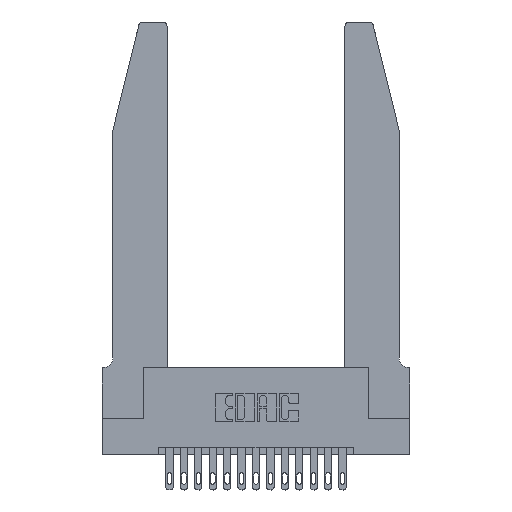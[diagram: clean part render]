
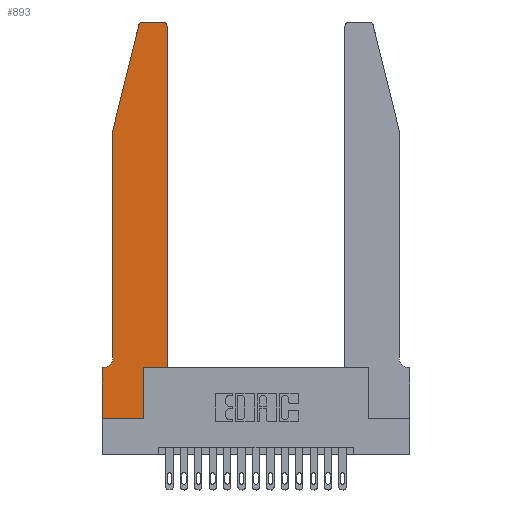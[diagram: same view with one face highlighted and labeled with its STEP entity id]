
A CAD part, top view. The second image highlights one B-rep face of the part: STEP entity #893.
In plain terms, the highlighted planar face has unit normal (0, 0, 1).
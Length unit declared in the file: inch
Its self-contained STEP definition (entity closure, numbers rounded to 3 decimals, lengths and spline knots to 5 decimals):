
#21 = EDGE_CURVE ( 'NONE', #11869, #1695, #6208, .T. ) ;
#676 = LINE ( 'NONE', #16125, #11830 ) ;
#682 = LINE ( 'NONE', #17284, #14336 ) ;
#893 = ADVANCED_FACE ( 'NONE', ( #14101 ), #13317, .T. ) ;
#1071 = EDGE_CURVE ( 'NONE', #3224, #1689, #9797, .T. ) ;
#1089 = LINE ( 'NONE', #2618, #12228 ) ;
#1237 = DIRECTION ( 'NONE',  ( 0., 0., 1. ) ) ;
#1266 = DIRECTION ( 'NONE',  ( -1., 0., 0. ) ) ;
#1309 = VERTEX_POINT ( 'NONE', #16686 ) ;
#1320 = CARTESIAN_POINT ( 'NONE',  ( 0.2865, 0., 0.37 ) ) ;
#1689 = VERTEX_POINT ( 'NONE', #12186 ) ;
#1695 = VERTEX_POINT ( 'NONE', #10525 ) ;
#1908 = ORIENTED_EDGE ( 'NONE', *, *, #2524, .T. ) ;
#2524 = EDGE_CURVE ( 'NONE', #1309, #9897, #1089, .T. ) ;
#2617 = EDGE_CURVE ( 'NONE', #15138, #11822, #16069, .T. ) ;
#2618 = CARTESIAN_POINT ( 'NONE',  ( 0.4505, 0.35, 0.37 ) ) ;
#2886 = VECTOR ( 'NONE', #10107, 39.37008 ) ;
#2991 = CARTESIAN_POINT ( 'NONE',  ( 0.4505, 0.35, 0.37 ) ) ;
#3032 = ORIENTED_EDGE ( 'NONE', *, *, #14612, .T. ) ;
#3224 = VERTEX_POINT ( 'NONE', #11714 ) ;
#3293 = VECTOR ( 'NONE', #7868, 39.37008 ) ;
#3381 = DIRECTION ( 'NONE',  ( 0., 0., 1. ) ) ;
#3836 = EDGE_CURVE ( 'NONE', #9897, #15138, #10806, .T. ) ;
#3841 = EDGE_CURVE ( 'NONE', #11676, #11869, #8314, .T. ) ;
#3956 = CARTESIAN_POINT ( 'NONE',  ( 0.2605, 2.75, 0.37 ) ) ;
#4346 = VERTEX_POINT ( 'NONE', #6788 ) ;
#4356 = CARTESIAN_POINT ( 'NONE',  ( 0.0055, 0.42, 0.37 ) ) ;
#5169 = CARTESIAN_POINT ( 'NONE',  ( 0.0755, 2., 0.37 ) ) ;
#5445 = ORIENTED_EDGE ( 'NONE', *, *, #11831, .T. ) ;
#5540 = DIRECTION ( 'NONE',  ( 1., 0., 0. ) ) ;
#5554 = DIRECTION ( 'NONE',  ( 0., -1., 0. ) ) ;
#5788 = AXIS2_PLACEMENT_3D ( 'NONE', #11943, #3381, #10596 ) ;
#5936 = VECTOR ( 'NONE', #10603, 39.37008 ) ;
#6208 = CIRCLE ( 'NONE', #13917, 0.07 ) ;
#6650 = CARTESIAN_POINT ( 'NONE',  ( 0.0755, 2., 0.37 ) ) ;
#6704 = EDGE_LOOP ( 'NONE', ( #5445, #10141, #14673, #13111, #17718, #12790, #18360, #12419, #3032, #1908, #17313, #9536 ) ) ;
#6788 = CARTESIAN_POINT ( 'NONE',  ( 0.284, 2.75, 0.37 ) ) ;
#7584 = DIRECTION ( 'NONE',  ( 1., 0., 0. ) ) ;
#7868 = DIRECTION ( 'NONE',  ( 0., 1., 0. ) ) ;
#7995 = DIRECTION ( 'NONE',  ( -0.239, -0.971, 0. ) ) ;
#8314 = LINE ( 'NONE', #18711, #11060 ) ;
#8891 = DIRECTION ( 'NONE',  ( 1., 0., 0. ) ) ;
#9236 = EDGE_CURVE ( 'NONE', #17259, #11676, #10289, .T. ) ;
#9365 = VECTOR ( 'NONE', #7995, 39.37008 ) ;
#9536 = ORIENTED_EDGE ( 'NONE', *, *, #2617, .T. ) ;
#9797 = LINE ( 'NONE', #16319, #5936 ) ;
#9897 = VERTEX_POINT ( 'NONE', #2991 ) ;
#9936 = VERTEX_POINT ( 'NONE', #1320 ) ;
#10107 = DIRECTION ( 'NONE',  ( 0., 1., 0. ) ) ;
#10141 = ORIENTED_EDGE ( 'NONE', *, *, #15587, .T. ) ;
#10289 = LINE ( 'NONE', #5169, #9365 ) ;
#10404 = DIRECTION ( 'NONE',  ( 0., 0., 1. ) ) ;
#10525 = CARTESIAN_POINT ( 'NONE',  ( 0.0055, 0.35, 0.37 ) ) ;
#10537 = CARTESIAN_POINT ( 'NONE',  ( 0.4505, 2.72, 0.37 ) ) ;
#10596 = DIRECTION ( 'NONE',  ( 1., 0., 0. ) ) ;
#10603 = DIRECTION ( 'NONE',  ( 0., -1., 0. ) ) ;
#10806 = LINE ( 'NONE', #11510, #2886 ) ;
#11017 = EDGE_CURVE ( 'NONE', #1695, #3224, #682, .T. ) ;
#11060 = VECTOR ( 'NONE', #5554, 39.37008 ) ;
#11303 = CARTESIAN_POINT ( 'NONE',  ( 0.4205, 2.75, 0.37 ) ) ;
#11510 = CARTESIAN_POINT ( 'NONE',  ( 0.4505, 0.35, 0.37 ) ) ;
#11676 = VERTEX_POINT ( 'NONE', #6650 ) ;
#11714 = CARTESIAN_POINT ( 'NONE',  ( 0., 0.35, 0.37 ) ) ;
#11822 = VERTEX_POINT ( 'NONE', #11303 ) ;
#11830 = VECTOR ( 'NONE', #8891, 39.37008 ) ;
#11831 = EDGE_CURVE ( 'NONE', #11822, #4346, #12698, .T. ) ;
#11869 = VERTEX_POINT ( 'NONE', #12575 ) ;
#11943 = CARTESIAN_POINT ( 'NONE',  ( 0., 0.35, 0.37 ) ) ;
#12186 = CARTESIAN_POINT ( 'NONE',  ( 0., 0., 0.37 ) ) ;
#12228 = VECTOR ( 'NONE', #5540, 39.37008 ) ;
#12419 = ORIENTED_EDGE ( 'NONE', *, *, #16807, .T. ) ;
#12575 = CARTESIAN_POINT ( 'NONE',  ( 0.0755, 0.42, 0.37 ) ) ;
#12698 = LINE ( 'NONE', #3956, #12942 ) ;
#12790 = ORIENTED_EDGE ( 'NONE', *, *, #11017, .T. ) ;
#12942 = VECTOR ( 'NONE', #14205, 39.37008 ) ;
#13111 = ORIENTED_EDGE ( 'NONE', *, *, #3841, .T. ) ;
#13317 = PLANE ( 'NONE',  #5788 ) ;
#13917 = AXIS2_PLACEMENT_3D ( 'NONE', #4356, #17276, #18707 ) ;
#14101 = FACE_OUTER_BOUND ( 'NONE', #6704, .T. ) ;
#14205 = DIRECTION ( 'NONE',  ( -1., 0., 0. ) ) ;
#14336 = VECTOR ( 'NONE', #1266, 39.37008 ) ;
#14352 = CARTESIAN_POINT ( 'NONE',  ( 0.4205, 2.72, 0.37 ) ) ;
#14388 = CIRCLE ( 'NONE', #14702, 0.03 ) ;
#14612 = EDGE_CURVE ( 'NONE', #9936, #1309, #17141, .T. ) ;
#14673 = ORIENTED_EDGE ( 'NONE', *, *, #9236, .T. ) ;
#14702 = AXIS2_PLACEMENT_3D ( 'NONE', #17379, #1237, #17260 ) ;
#15138 = VERTEX_POINT ( 'NONE', #10537 ) ;
#15450 = CARTESIAN_POINT ( 'NONE',  ( 0.25487, 2.72718, 0.37 ) ) ;
#15539 = AXIS2_PLACEMENT_3D ( 'NONE', #14352, #10404, #7584 ) ;
#15587 = EDGE_CURVE ( 'NONE', #4346, #17259, #14388, .T. ) ;
#16069 = CIRCLE ( 'NONE', #15539, 0.03 ) ;
#16125 = CARTESIAN_POINT ( 'NONE',  ( 0., 0., 0.37 ) ) ;
#16319 = CARTESIAN_POINT ( 'NONE',  ( 0., 0., 0.37 ) ) ;
#16686 = CARTESIAN_POINT ( 'NONE',  ( 0.2865, 0.35, 0.37 ) ) ;
#16807 = EDGE_CURVE ( 'NONE', #1689, #9936, #676, .T. ) ;
#17141 = LINE ( 'NONE', #17979, #3293 ) ;
#17259 = VERTEX_POINT ( 'NONE', #15450 ) ;
#17260 = DIRECTION ( 'NONE',  ( 1., 0., 0. ) ) ;
#17276 = DIRECTION ( 'NONE',  ( 0., 0., -1. ) ) ;
#17284 = CARTESIAN_POINT ( 'NONE',  ( 0.0755, 0.35, 0.37 ) ) ;
#17313 = ORIENTED_EDGE ( 'NONE', *, *, #3836, .T. ) ;
#17379 = CARTESIAN_POINT ( 'NONE',  ( 0.284, 2.72, 0.37 ) ) ;
#17718 = ORIENTED_EDGE ( 'NONE', *, *, #21, .T. ) ;
#17979 = CARTESIAN_POINT ( 'NONE',  ( 0.2865, 0.35, 0.37 ) ) ;
#18360 = ORIENTED_EDGE ( 'NONE', *, *, #1071, .T. ) ;
#18707 = DIRECTION ( 'NONE',  ( -1., 0., 0. ) ) ;
#18711 = CARTESIAN_POINT ( 'NONE',  ( 0.0755, 2., 0.37 ) ) ;
